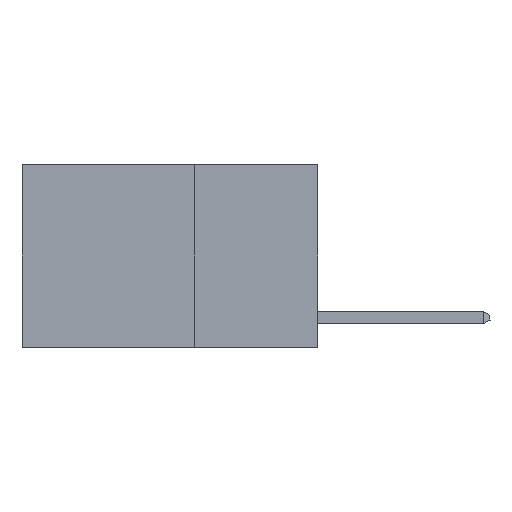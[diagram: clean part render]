
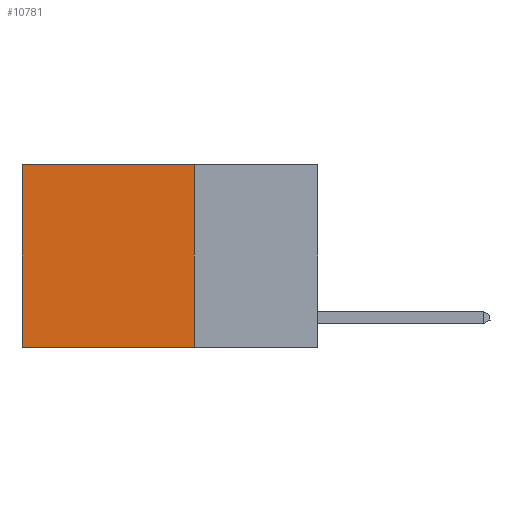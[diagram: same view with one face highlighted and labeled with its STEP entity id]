
A CAD part, left-side view. The second image highlights one B-rep face of the part: STEP entity #10781.
In plain terms, the highlighted planar face has unit normal (-1, 0, 0).
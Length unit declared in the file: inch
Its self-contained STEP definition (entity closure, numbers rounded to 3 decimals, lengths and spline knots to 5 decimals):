
#396 = LINE ( 'NONE', #6256, #4494 ) ;
#445 = DIRECTION ( 'NONE',  ( 1., 0., 0. ) ) ;
#973 = EDGE_CURVE ( 'NONE', #16916, #16215, #17637, .T. ) ;
#1431 = EDGE_CURVE ( 'NONE', #16230, #6876, #396, .T. ) ;
#1606 = LINE ( 'NONE', #1678, #8525 ) ;
#1678 = CARTESIAN_POINT ( 'NONE',  ( 0.2625, 0.6, 0. ) ) ;
#2309 = CARTESIAN_POINT ( 'NONE',  ( 0.2625, 0.25, -0.37 ) ) ;
#2597 = AXIS2_PLACEMENT_3D ( 'NONE', #16903, #445, #10046 ) ;
#2660 = EDGE_CURVE ( 'NONE', #16230, #16916, #5736, .T. ) ;
#3096 = EDGE_CURVE ( 'NONE', #6876, #16215, #1606, .T. ) ;
#3442 = ORIENTED_EDGE ( 'NONE', *, *, #1431, .T. ) ;
#4471 = DIRECTION ( 'NONE',  ( 0., 0., -1. ) ) ;
#4494 = VECTOR ( 'NONE', #8960, 39.37008 ) ;
#4902 = CARTESIAN_POINT ( 'NONE',  ( 0.2625, 0.25, 0. ) ) ;
#4996 = EDGE_LOOP ( 'NONE', ( #8286, #13846, #6742, #3442 ) ) ;
#5285 = FACE_OUTER_BOUND ( 'NONE', #4996, .T. ) ;
#5513 = DIRECTION ( 'NONE',  ( 0., 1., 0. ) ) ;
#5736 = LINE ( 'NONE', #4902, #16252 ) ;
#6256 = CARTESIAN_POINT ( 'NONE',  ( 0.2625, 0.25, 0. ) ) ;
#6675 = VECTOR ( 'NONE', #5513, 39.37008 ) ;
#6742 = ORIENTED_EDGE ( 'NONE', *, *, #2660, .F. ) ;
#6876 = VERTEX_POINT ( 'NONE', #15273 ) ;
#7317 = PLANE ( 'NONE',  #2597 ) ;
#8286 = ORIENTED_EDGE ( 'NONE', *, *, #3096, .T. ) ;
#8525 = VECTOR ( 'NONE', #4471, 39.37008 ) ;
#8960 = DIRECTION ( 'NONE',  ( 0., 1., 0. ) ) ;
#9441 = CARTESIAN_POINT ( 'NONE',  ( 0.2625, 0.6, -0.37 ) ) ;
#10046 = DIRECTION ( 'NONE',  ( 0., 0., -1. ) ) ;
#10781 = ADVANCED_FACE ( 'NONE', ( #5285 ), #7317, .F. ) ;
#12183 = CARTESIAN_POINT ( 'NONE',  ( 0.2625, 0.25, 0. ) ) ;
#13846 = ORIENTED_EDGE ( 'NONE', *, *, #973, .F. ) ;
#15273 = CARTESIAN_POINT ( 'NONE',  ( 0.2625, 0.6, 0. ) ) ;
#15878 = DIRECTION ( 'NONE',  ( 0., 0., -1. ) ) ;
#16215 = VERTEX_POINT ( 'NONE', #9441 ) ;
#16230 = VERTEX_POINT ( 'NONE', #12183 ) ;
#16252 = VECTOR ( 'NONE', #15878, 39.37008 ) ;
#16628 = CARTESIAN_POINT ( 'NONE',  ( 0.2625, 0.25, -0.37 ) ) ;
#16903 = CARTESIAN_POINT ( 'NONE',  ( 0.2625, 0.25, 0. ) ) ;
#16916 = VERTEX_POINT ( 'NONE', #16628 ) ;
#17637 = LINE ( 'NONE', #2309, #6675 ) ;
